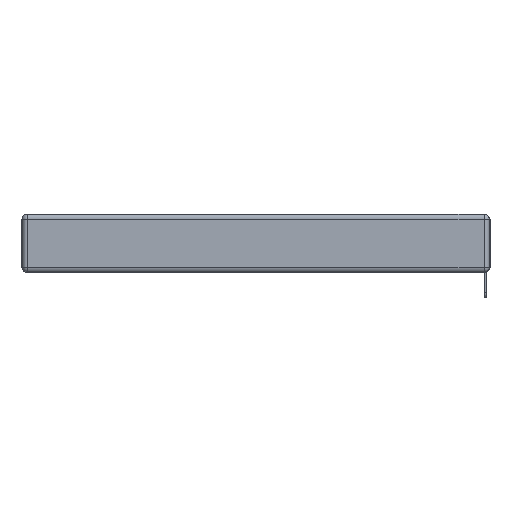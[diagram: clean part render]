
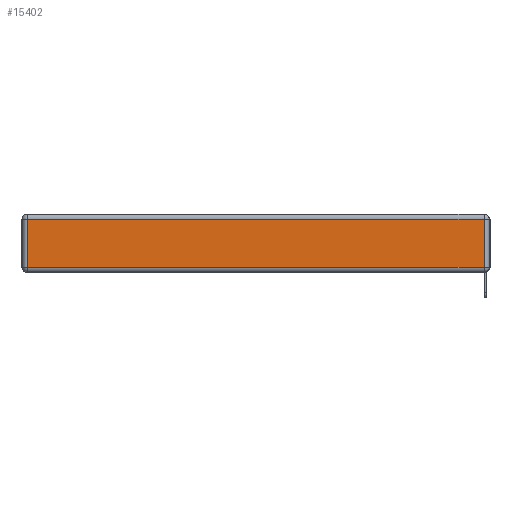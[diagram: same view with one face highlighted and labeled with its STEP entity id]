
A CAD part, left-side view. The second image highlights one B-rep face of the part: STEP entity #15402.
In plain terms, the highlighted planar face has unit normal (-1, 0, 0).
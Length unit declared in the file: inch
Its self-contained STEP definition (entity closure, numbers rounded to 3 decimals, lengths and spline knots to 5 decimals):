
#411 = DIRECTION ( 'NONE',  ( 0., 0., -1. ) ) ;
#471 = CARTESIAN_POINT ( 'NONE',  ( 0., 2.72, -0.03 ) ) ;
#766 = CARTESIAN_POINT ( 'NONE',  ( 0., 0.03, -0.313 ) ) ;
#1574 = EDGE_CURVE ( 'NONE', #4216, #11085, #9734, .T. ) ;
#2832 = ORIENTED_EDGE ( 'NONE', *, *, #6673, .T. ) ;
#2987 = CARTESIAN_POINT ( 'NONE',  ( 0., 0.03, -0.343 ) ) ;
#3675 = LINE ( 'NONE', #10204, #5509 ) ;
#4038 = PLANE ( 'NONE',  #17352 ) ;
#4216 = VERTEX_POINT ( 'NONE', #4840 ) ;
#4654 = VECTOR ( 'NONE', #12854, 39.37008 ) ;
#4840 = CARTESIAN_POINT ( 'NONE',  ( 0., 0.03, -0.03 ) ) ;
#5304 = VECTOR ( 'NONE', #411, 39.37008 ) ;
#5362 = EDGE_LOOP ( 'NONE', ( #5805, #9939, #8504, #2832 ) ) ;
#5509 = VECTOR ( 'NONE', #17357, 39.37008 ) ;
#5805 = ORIENTED_EDGE ( 'NONE', *, *, #7906, .T. ) ;
#6673 = EDGE_CURVE ( 'NONE', #11085, #14451, #13724, .T. ) ;
#7906 = EDGE_CURVE ( 'NONE', #14451, #17268, #3675, .T. ) ;
#8487 = CARTESIAN_POINT ( 'NONE',  ( 0., 2.75, -0.03 ) ) ;
#8504 = ORIENTED_EDGE ( 'NONE', *, *, #1574, .T. ) ;
#9734 = LINE ( 'NONE', #8487, #15689 ) ;
#9939 = ORIENTED_EDGE ( 'NONE', *, *, #16055, .T. ) ;
#10204 = CARTESIAN_POINT ( 'NONE',  ( 0., 0., -0.313 ) ) ;
#11085 = VERTEX_POINT ( 'NONE', #471 ) ;
#12003 = FACE_OUTER_BOUND ( 'NONE', #5362, .T. ) ;
#12473 = DIRECTION ( 'NONE',  ( -1., 0., 0. ) ) ;
#12854 = DIRECTION ( 'NONE',  ( 0., 0., 1. ) ) ;
#13724 = LINE ( 'NONE', #15914, #5304 ) ;
#14044 = DIRECTION ( 'NONE',  ( 0., 0., 1. ) ) ;
#14429 = LINE ( 'NONE', #2987, #4654 ) ;
#14451 = VERTEX_POINT ( 'NONE', #17412 ) ;
#15346 = CARTESIAN_POINT ( 'NONE',  ( 0., 0., -0.343 ) ) ;
#15402 = ADVANCED_FACE ( 'NONE', ( #12003 ), #4038, .T. ) ;
#15689 = VECTOR ( 'NONE', #15889, 39.37008 ) ;
#15889 = DIRECTION ( 'NONE',  ( 0., 1., 0. ) ) ;
#15914 = CARTESIAN_POINT ( 'NONE',  ( 0., 2.72, -0.343 ) ) ;
#16055 = EDGE_CURVE ( 'NONE', #17268, #4216, #14429, .T. ) ;
#17268 = VERTEX_POINT ( 'NONE', #766 ) ;
#17352 = AXIS2_PLACEMENT_3D ( 'NONE', #15346, #12473, #14044 ) ;
#17357 = DIRECTION ( 'NONE',  ( 0., -1., 0. ) ) ;
#17412 = CARTESIAN_POINT ( 'NONE',  ( 0., 2.72, -0.313 ) ) ;
